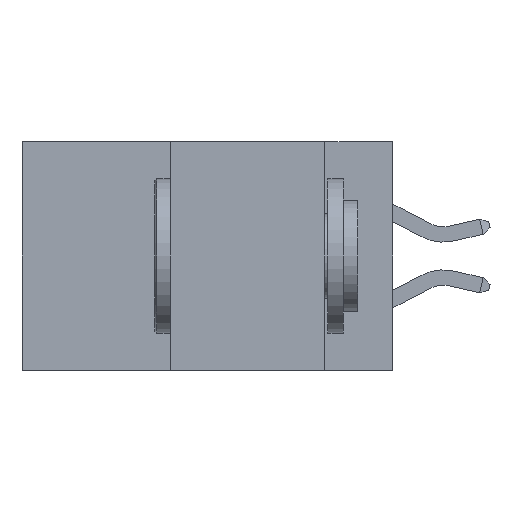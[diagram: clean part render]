
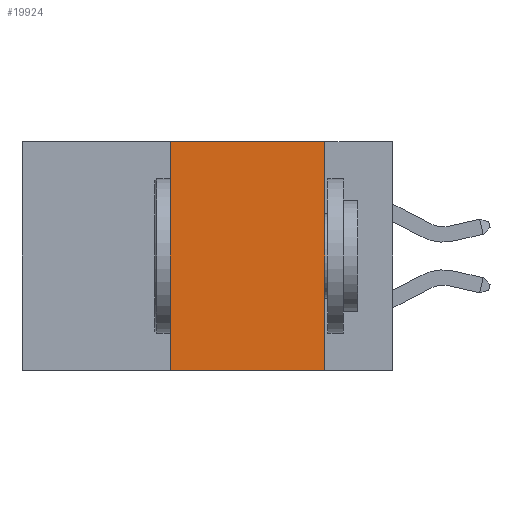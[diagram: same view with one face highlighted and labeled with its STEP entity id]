
A CAD part, left-side view. The second image highlights one B-rep face of the part: STEP entity #19924.
In plain terms, the highlighted planar face has unit normal (-1, 0, 0).
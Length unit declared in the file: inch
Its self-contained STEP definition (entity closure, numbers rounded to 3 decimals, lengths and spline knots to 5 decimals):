
#597 = CARTESIAN_POINT ( 'NONE',  ( 0., 0.11, -0.37 ) ) ;
#1757 = AXIS2_PLACEMENT_3D ( 'NONE', #17993, #19773, #8989 ) ;
#3561 = CARTESIAN_POINT ( 'NONE',  ( 0., 0.36, 0. ) ) ;
#3631 = CARTESIAN_POINT ( 'NONE',  ( 0., 0.11, 0. ) ) ;
#5337 = PLANE ( 'NONE',  #1757 ) ;
#5357 = VECTOR ( 'NONE', #18090, 39.37008 ) ;
#5857 = VERTEX_POINT ( 'NONE', #7043 ) ;
#5984 = ORIENTED_EDGE ( 'NONE', *, *, #7665, .F. ) ;
#6288 = VERTEX_POINT ( 'NONE', #11876 ) ;
#6503 = LINE ( 'NONE', #3561, #5357 ) ;
#7043 = CARTESIAN_POINT ( 'NONE',  ( 0., 0.36, -0.37 ) ) ;
#7127 = ORIENTED_EDGE ( 'NONE', *, *, #13731, .F. ) ;
#7333 = DIRECTION ( 'NONE',  ( 0., 0., -1. ) ) ;
#7665 = EDGE_CURVE ( 'NONE', #6288, #11568, #23354, .T. ) ;
#7707 = ORIENTED_EDGE ( 'NONE', *, *, #11309, .T. ) ;
#7742 = EDGE_LOOP ( 'NONE', ( #5984, #16186, #7127, #7707 ) ) ;
#8267 = LINE ( 'NONE', #12794, #17303 ) ;
#8989 = DIRECTION ( 'NONE',  ( 0., 0., -1. ) ) ;
#9457 = LINE ( 'NONE', #19922, #18491 ) ;
#9904 = VERTEX_POINT ( 'NONE', #22664 ) ;
#10967 = DIRECTION ( 'NONE',  ( 0., -1., 0. ) ) ;
#11309 = EDGE_CURVE ( 'NONE', #5857, #11568, #9457, .T. ) ;
#11568 = VERTEX_POINT ( 'NONE', #597 ) ;
#11876 = CARTESIAN_POINT ( 'NONE',  ( 0., 0.11, 0. ) ) ;
#12794 = CARTESIAN_POINT ( 'NONE',  ( 0., 0.6, 0. ) ) ;
#13731 = EDGE_CURVE ( 'NONE', #5857, #9904, #6503, .T. ) ;
#16186 = ORIENTED_EDGE ( 'NONE', *, *, #19979, .F. ) ;
#17303 = VECTOR ( 'NONE', #23493, 39.37008 ) ;
#17993 = CARTESIAN_POINT ( 'NONE',  ( 0., 0.6, 0. ) ) ;
#18090 = DIRECTION ( 'NONE',  ( 0., 0., 1. ) ) ;
#18491 = VECTOR ( 'NONE', #10967, 39.37008 ) ;
#18631 = VECTOR ( 'NONE', #7333, 39.37008 ) ;
#19773 = DIRECTION ( 'NONE',  ( 1., 0., 0. ) ) ;
#19922 = CARTESIAN_POINT ( 'NONE',  ( 0., 0.6, -0.37 ) ) ;
#19924 = ADVANCED_FACE ( 'NONE', ( #23166 ), #5337, .F. ) ;
#19979 = EDGE_CURVE ( 'NONE', #9904, #6288, #8267, .T. ) ;
#22664 = CARTESIAN_POINT ( 'NONE',  ( 0., 0.36, 0. ) ) ;
#23166 = FACE_OUTER_BOUND ( 'NONE', #7742, .T. ) ;
#23354 = LINE ( 'NONE', #3631, #18631 ) ;
#23493 = DIRECTION ( 'NONE',  ( 0., -1., 0. ) ) ;
